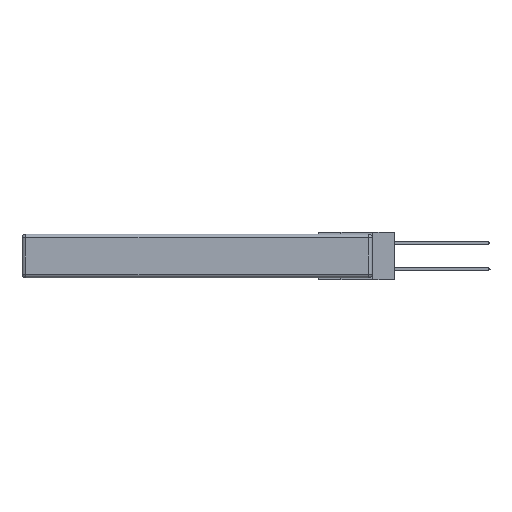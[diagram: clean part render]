
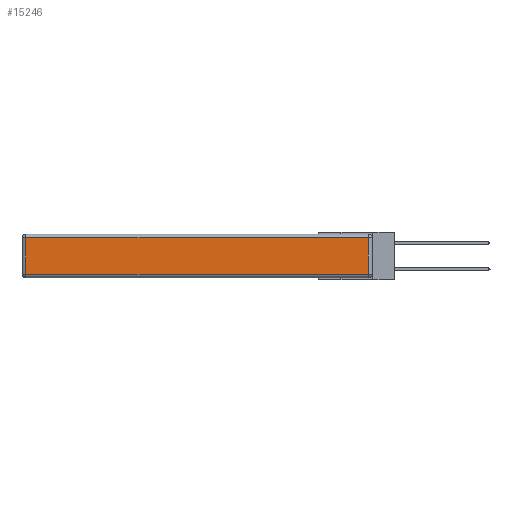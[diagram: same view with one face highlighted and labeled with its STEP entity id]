
A CAD part, left-side view. The second image highlights one B-rep face of the part: STEP entity #15246.
In plain terms, the highlighted planar face has unit normal (-1, 0, 0).
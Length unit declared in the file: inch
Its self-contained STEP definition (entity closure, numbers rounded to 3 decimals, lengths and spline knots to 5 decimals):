
#60 = EDGE_LOOP ( 'NONE', ( #11322, #12278, #14983, #4701 ) ) ;
#262 = CARTESIAN_POINT ( 'NONE',  ( 0., 2.72, -0.03 ) ) ;
#332 = CARTESIAN_POINT ( 'NONE',  ( 0., 2.72, -0.343 ) ) ;
#806 = EDGE_CURVE ( 'NONE', #12983, #5951, #15242, .T. ) ;
#1235 = CARTESIAN_POINT ( 'NONE',  ( 0., 0., -0.313 ) ) ;
#1343 = CARTESIAN_POINT ( 'NONE',  ( 0., 2.72, -0.313 ) ) ;
#1574 = LINE ( 'NONE', #8643, #7527 ) ;
#1617 = VECTOR ( 'NONE', #15185, 39.37008 ) ;
#1741 = CARTESIAN_POINT ( 'NONE',  ( 0., 0.03, -0.313 ) ) ;
#2226 = DIRECTION ( 'NONE',  ( 0., 0., 1. ) ) ;
#4149 = PLANE ( 'NONE',  #8719 ) ;
#4701 = ORIENTED_EDGE ( 'NONE', *, *, #806, .T. ) ;
#5698 = VERTEX_POINT ( 'NONE', #6093 ) ;
#5951 = VERTEX_POINT ( 'NONE', #1343 ) ;
#6093 = CARTESIAN_POINT ( 'NONE',  ( 0., 0.03, -0.03 ) ) ;
#6558 = EDGE_CURVE ( 'NONE', #11930, #5698, #13381, .T. ) ;
#6991 = CARTESIAN_POINT ( 'NONE',  ( 0., 0.03, -0.343 ) ) ;
#7246 = VECTOR ( 'NONE', #2226, 39.37008 ) ;
#7527 = VECTOR ( 'NONE', #11128, 39.37008 ) ;
#8643 = CARTESIAN_POINT ( 'NONE',  ( 0., 2.75, -0.03 ) ) ;
#8719 = AXIS2_PLACEMENT_3D ( 'NONE', #15298, #12694, #9023 ) ;
#9023 = DIRECTION ( 'NONE',  ( 0., 0., 1. ) ) ;
#9988 = EDGE_CURVE ( 'NONE', #5698, #12983, #1574, .T. ) ;
#11128 = DIRECTION ( 'NONE',  ( 0., 1., 0. ) ) ;
#11322 = ORIENTED_EDGE ( 'NONE', *, *, #14885, .T. ) ;
#11776 = VECTOR ( 'NONE', #13500, 39.37008 ) ;
#11930 = VERTEX_POINT ( 'NONE', #1741 ) ;
#12278 = ORIENTED_EDGE ( 'NONE', *, *, #6558, .T. ) ;
#12694 = DIRECTION ( 'NONE',  ( -1., 0., 0. ) ) ;
#12983 = VERTEX_POINT ( 'NONE', #262 ) ;
#13381 = LINE ( 'NONE', #6991, #7246 ) ;
#13500 = DIRECTION ( 'NONE',  ( 0., -1., 0. ) ) ;
#14027 = FACE_OUTER_BOUND ( 'NONE', #60, .T. ) ;
#14885 = EDGE_CURVE ( 'NONE', #5951, #11930, #15802, .T. ) ;
#14983 = ORIENTED_EDGE ( 'NONE', *, *, #9988, .T. ) ;
#15185 = DIRECTION ( 'NONE',  ( 0., 0., -1. ) ) ;
#15242 = LINE ( 'NONE', #332, #1617 ) ;
#15246 = ADVANCED_FACE ( 'NONE', ( #14027 ), #4149, .T. ) ;
#15298 = CARTESIAN_POINT ( 'NONE',  ( 0., 0., -0.343 ) ) ;
#15802 = LINE ( 'NONE', #1235, #11776 ) ;
